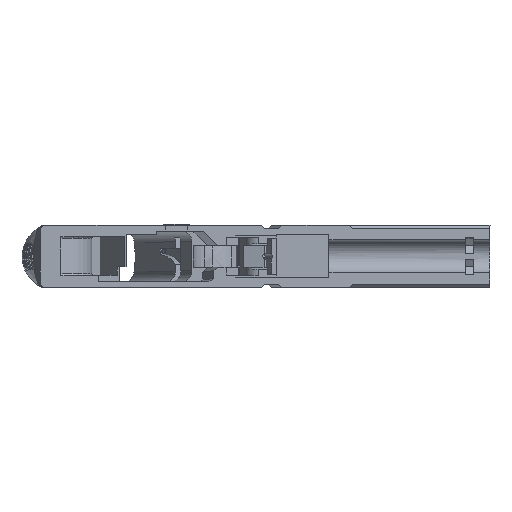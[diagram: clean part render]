
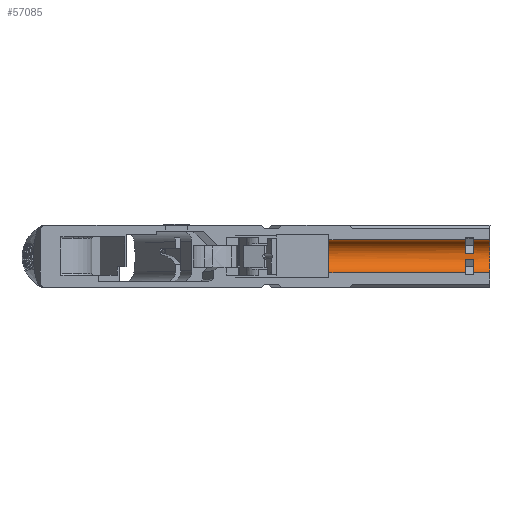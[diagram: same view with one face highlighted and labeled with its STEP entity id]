
A CAD part, top view. The second image highlights one B-rep face of the part: STEP entity #57085.
In plain terms, the highlighted free-form (B-spline) face has degree [1, 2] with [2, 5] control points.
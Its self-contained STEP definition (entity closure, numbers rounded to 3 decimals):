
#3908=(
BOUNDED_SURFACE()
B_SPLINE_SURFACE(1,2,((#68974,#68975,#68976,#68977,#68978),(#68979,#68980,
#68981,#68982,#68983)),.UNSPECIFIED.,.F.,.F.,.F.)
B_SPLINE_SURFACE_WITH_KNOTS((2,2),(3,2,3),(-9.79,-0.013),
(-1.554,0.,1.554),.UNSPECIFIED.)
GEOMETRIC_REPRESENTATION_ITEM()
RATIONAL_B_SPLINE_SURFACE(((1.,0.713,1.,0.713,1.),
(1.,0.713,1.,0.713,1.)))
REPRESENTATION_ITEM('')
SURFACE()
);
#8873=FACE_OUTER_BOUND('',#12323,.T.);
#12323=EDGE_LOOP('',(#39225,#39226,#39227,#39228,#39229,#39230,#39231,#39232,
#39233,#39234,#39235,#39236));
#16349=LINE('',#68908,#20112);
#16366=LINE('',#68947,#20129);
#16367=LINE('',#68949,#20130);
#16378=LINE('',#68985,#20141);
#16379=LINE('',#68989,#20142);
#16380=LINE('',#68992,#20143);
#20112=VECTOR('',#62161,7.765);
#20129=VECTOR('',#62194,10.);
#20130=VECTOR('',#62197,10.);
#20141=VECTOR('',#62220,7.765);
#20142=VECTOR('',#62223,7.765);
#20143=VECTOR('',#62226,10.);
#23706=CIRCLE('',#60507,7.765);
#23709=CIRCLE('',#60536,7.765);
#23710=CIRCLE('',#60540,7.765);
#23712=CIRCLE('',#60545,7.765);
#23714=CIRCLE('',#60550,7.765);
#23715=CIRCLE('',#60551,7.765);
#23988=VERTEX_POINT('',#68625);
#23989=VERTEX_POINT('',#68627);
#24085=VERTEX_POINT('',#68906);
#24086=VERTEX_POINT('',#68910);
#24087=VERTEX_POINT('',#68911);
#24096=VERTEX_POINT('',#68936);
#24097=VERTEX_POINT('',#68938);
#24102=VERTEX_POINT('',#68955);
#24108=VERTEX_POINT('',#68984);
#24109=VERTEX_POINT('',#68986);
#24110=VERTEX_POINT('',#68988);
#24111=VERTEX_POINT('',#68990);
#29964=EDGE_CURVE('',#23989,#23988,#23706,.T.);
#30087=EDGE_CURVE('',#24085,#23989,#16349,.T.);
#30088=EDGE_CURVE('',#24086,#24087,#23709,.F.);
#30102=EDGE_CURVE('',#24097,#24096,#23710,.T.);
#30107=EDGE_CURVE('',#24097,#23988,#16366,.T.);
#30108=EDGE_CURVE('',#24087,#24096,#16367,.T.);
#30111=EDGE_CURVE('',#24102,#24085,#23712,.T.);
#30121=EDGE_CURVE('',#24108,#24086,#16378,.T.);
#30122=EDGE_CURVE('',#24108,#24109,#23714,.T.);
#30123=EDGE_CURVE('',#24109,#24110,#16379,.T.);
#30124=EDGE_CURVE('',#24110,#24111,#23715,.T.);
#30125=EDGE_CURVE('',#24111,#24102,#16380,.T.);
#39225=ORIENTED_EDGE('',*,*,#29964,.T.);
#39226=ORIENTED_EDGE('',*,*,#30107,.F.);
#39227=ORIENTED_EDGE('',*,*,#30102,.T.);
#39228=ORIENTED_EDGE('',*,*,#30108,.F.);
#39229=ORIENTED_EDGE('',*,*,#30088,.F.);
#39230=ORIENTED_EDGE('',*,*,#30121,.F.);
#39231=ORIENTED_EDGE('',*,*,#30122,.T.);
#39232=ORIENTED_EDGE('',*,*,#30123,.T.);
#39233=ORIENTED_EDGE('',*,*,#30124,.T.);
#39234=ORIENTED_EDGE('',*,*,#30125,.T.);
#39235=ORIENTED_EDGE('',*,*,#30111,.T.);
#39236=ORIENTED_EDGE('',*,*,#30087,.T.);
#57085=ADVANCED_FACE('',(#8873),#3908,.T.);
#60507=AXIS2_PLACEMENT_3D('',#68628,#61991,#61992);
#60536=AXIS2_PLACEMENT_3D('',#68912,#62164,#62165);
#60540=AXIS2_PLACEMENT_3D('',#68939,#62185,#62186);
#60545=AXIS2_PLACEMENT_3D('',#68956,#62202,#62203);
#60550=AXIS2_PLACEMENT_3D('',#68987,#62221,#62222);
#60551=AXIS2_PLACEMENT_3D('',#68991,#62224,#62225);
#61991=DIRECTION('center_axis',(1.,0.,0.));
#61992=DIRECTION('ref_axis',(0.,0.,
-1.));
#62161=DIRECTION('',(1.,0.,0.));
#62164=DIRECTION('center_axis',(1.,0.,0.));
#62165=DIRECTION('ref_axis',(0.,0.,
-1.));
#62185=DIRECTION('center_axis',(-1.,0.,0.));
#62186=DIRECTION('ref_axis',(0.,0.,
-1.));
#62194=DIRECTION('',(1.,0.,0.));
#62197=DIRECTION('',(1.,0.,0.));
#62202=DIRECTION('center_axis',(-1.,0.,0.));
#62203=DIRECTION('ref_axis',(0.,0.,
-1.));
#62220=DIRECTION('',(1.,0.,0.));
#62221=DIRECTION('center_axis',(-1.,0.,0.));
#62222=DIRECTION('ref_axis',(0.,0.,
-1.));
#62223=DIRECTION('',(1.,0.,0.));
#62224=DIRECTION('center_axis',(1.,0.,0.));
#62225=DIRECTION('ref_axis',(0.,0.,
-1.));
#62226=DIRECTION('',(1.,0.,0.));
#68625=CARTESIAN_POINT('',(179.035,34.275,-265.477));
#68627=CARTESIAN_POINT('',(179.035,18.747,-265.477));
#68628=CARTESIAN_POINT('Origin',(179.035,26.511,-265.35));
#68906=CARTESIAN_POINT('',(171.385,18.747,-265.477));
#68908=CARTESIAN_POINT('',(179.135,18.747,-265.477));
#68910=CARTESIAN_POINT('',(167.385,34.275,-265.477));
#68911=CARTESIAN_POINT('',(167.385,28.047,-272.961));
#68912=CARTESIAN_POINT('Origin',(167.385,26.511,-265.35));
#68936=CARTESIAN_POINT('',(171.385,28.047,-272.961));
#68938=CARTESIAN_POINT('',(171.385,34.275,-265.477));
#68939=CARTESIAN_POINT('Origin',(171.385,26.511,-265.35));
#68947=CARTESIAN_POINT('',(134.135,34.275,-265.477));
#68949=CARTESIAN_POINT('',(179.135,28.047,-272.961));
#68955=CARTESIAN_POINT('',(171.385,24.975,-272.961));
#68956=CARTESIAN_POINT('Origin',(171.385,26.511,-265.35));
#68974=CARTESIAN_POINT('Ctrl Pts',(103.12,18.747,-265.477));
#68975=CARTESIAN_POINT('Ctrl Pts',(103.12,18.872,-273.115));
#68976=CARTESIAN_POINT('Ctrl Pts',(103.12,26.511,-273.115));
#68977=CARTESIAN_POINT('Ctrl Pts',(103.12,34.15,-273.115));
#68978=CARTESIAN_POINT('Ctrl Pts',(103.12,34.275,-265.477));
#68979=CARTESIAN_POINT('Ctrl Pts',(179.035,18.747,-265.477));
#68980=CARTESIAN_POINT('Ctrl Pts',(179.035,18.872,-273.115));
#68981=CARTESIAN_POINT('Ctrl Pts',(179.035,26.511,-273.115));
#68982=CARTESIAN_POINT('Ctrl Pts',(179.035,34.15,-273.115));
#68983=CARTESIAN_POINT('Ctrl Pts',(179.035,34.275,-265.477));
#68984=CARTESIAN_POINT('',(103.12,34.275,-265.477));
#68985=CARTESIAN_POINT('',(179.135,34.275,-265.477));
#68986=CARTESIAN_POINT('',(103.12,18.747,-265.477));
#68987=CARTESIAN_POINT('Origin',(103.12,26.511,-265.351));
#68988=CARTESIAN_POINT('',(167.385,18.747,-265.477));
#68989=CARTESIAN_POINT('',(158.135,18.747,-265.477));
#68990=CARTESIAN_POINT('',(167.385,24.975,-272.961));
#68991=CARTESIAN_POINT('Origin',(167.385,26.511,-265.35));
#68992=CARTESIAN_POINT('',(179.135,24.975,-272.961));
